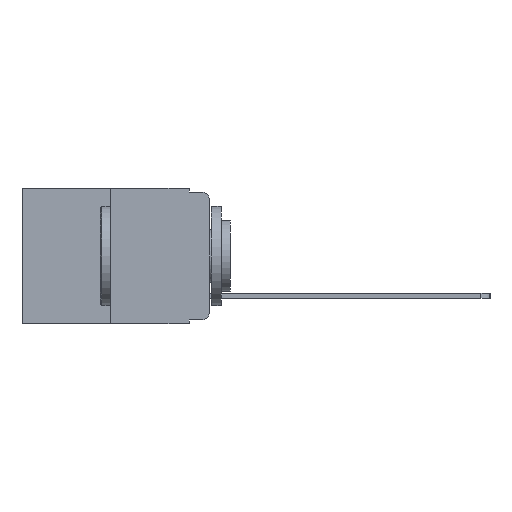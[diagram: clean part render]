
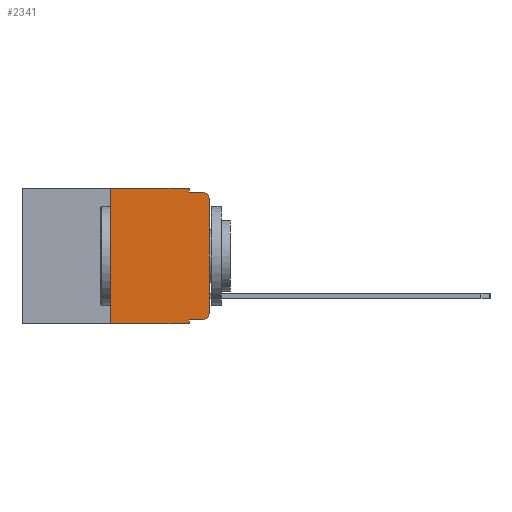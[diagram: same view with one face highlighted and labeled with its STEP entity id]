
A CAD part, left-side view. The second image highlights one B-rep face of the part: STEP entity #2341.
In plain terms, the highlighted planar face has unit normal (-1, 0, 0).
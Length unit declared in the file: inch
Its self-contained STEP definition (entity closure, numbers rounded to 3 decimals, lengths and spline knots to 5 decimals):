
#48 = CARTESIAN_POINT ( 'NONE',  ( 0., 0., -0.313 ) ) ;
#152 = LINE ( 'NONE', #20082, #4244 ) ;
#985 = CARTESIAN_POINT ( 'NONE',  ( 0., 0.25, 0. ) ) ;
#1154 = VERTEX_POINT ( 'NONE', #12719 ) ;
#1157 = EDGE_CURVE ( 'NONE', #9940, #8158, #12915, .T. ) ;
#1359 = VECTOR ( 'NONE', #15396, 39.37008 ) ;
#2341 = ADVANCED_FACE ( 'NONE', ( #12849 ), #18219, .F. ) ;
#2524 = ORIENTED_EDGE ( 'NONE', *, *, #1157, .T. ) ;
#2680 = DIRECTION ( 'NONE',  ( 0., -1., 0. ) ) ;
#2773 = EDGE_CURVE ( 'NONE', #5005, #10495, #17322, .T. ) ;
#3749 = ORIENTED_EDGE ( 'NONE', *, *, #14038, .F. ) ;
#3844 = VERTEX_POINT ( 'NONE', #15057 ) ;
#3892 = ORIENTED_EDGE ( 'NONE', *, *, #15682, .T. ) ;
#3919 = EDGE_LOOP ( 'NONE', ( #14781, #5084, #3749, #15264, #5722, #4393, #7224, #4700, #3892, #2524 ) ) ;
#4244 = VECTOR ( 'NONE', #7782, 39.37008 ) ;
#4262 = AXIS2_PLACEMENT_3D ( 'NONE', #7187, #18032, #8850 ) ;
#4393 = ORIENTED_EDGE ( 'NONE', *, *, #7287, .F. ) ;
#4700 = ORIENTED_EDGE ( 'NONE', *, *, #8414, .F. ) ;
#5005 = VERTEX_POINT ( 'NONE', #12021 ) ;
#5084 = ORIENTED_EDGE ( 'NONE', *, *, #20448, .T. ) ;
#5722 = ORIENTED_EDGE ( 'NONE', *, *, #17112, .F. ) ;
#6088 = LINE ( 'NONE', #13974, #17572 ) ;
#7130 = CARTESIAN_POINT ( 'NONE',  ( 0., 0.051, -0.01 ) ) ;
#7187 = CARTESIAN_POINT ( 'NONE',  ( 0., 0.02, -0.03 ) ) ;
#7224 = ORIENTED_EDGE ( 'NONE', *, *, #13374, .T. ) ;
#7287 = EDGE_CURVE ( 'NONE', #1154, #10195, #15985, .T. ) ;
#7782 = DIRECTION ( 'NONE',  ( 0., 0., -1. ) ) ;
#8158 = VERTEX_POINT ( 'NONE', #48 ) ;
#8163 = CARTESIAN_POINT ( 'NONE',  ( 0., 0., -0.03 ) ) ;
#8414 = EDGE_CURVE ( 'NONE', #10343, #12757, #152, .T. ) ;
#8566 = CARTESIAN_POINT ( 'NONE',  ( 0., 0.473, 0. ) ) ;
#8850 = DIRECTION ( 'NONE',  ( 0., 0., -1. ) ) ;
#9265 = VECTOR ( 'NONE', #10903, 39.37008 ) ;
#9369 = DIRECTION ( 'NONE',  ( 0., -1., 0. ) ) ;
#9417 = DIRECTION ( 'NONE',  ( 0., 0., -1. ) ) ;
#9788 = LINE ( 'NONE', #19992, #9265 ) ;
#9876 = VECTOR ( 'NONE', #9369, 39.37008 ) ;
#9940 = VERTEX_POINT ( 'NONE', #15331 ) ;
#10195 = VERTEX_POINT ( 'NONE', #15844 ) ;
#10343 = VERTEX_POINT ( 'NONE', #19184 ) ;
#10495 = VERTEX_POINT ( 'NONE', #7130 ) ;
#10903 = DIRECTION ( 'NONE',  ( 0., -1., 0. ) ) ;
#11580 = CARTESIAN_POINT ( 'NONE',  ( 0., 0., 0. ) ) ;
#11679 = DIRECTION ( 'NONE',  ( 0., 0., -1. ) ) ;
#11693 = CIRCLE ( 'NONE', #4262, 0.02 ) ;
#11727 = DIRECTION ( 'NONE',  ( -1., 0., 0. ) ) ;
#11831 = CARTESIAN_POINT ( 'NONE',  ( 0., 0.02, -0.313 ) ) ;
#12021 = CARTESIAN_POINT ( 'NONE',  ( 0., 0.051, 0. ) ) ;
#12719 = CARTESIAN_POINT ( 'NONE',  ( 0., 0.25, -0.343 ) ) ;
#12757 = VERTEX_POINT ( 'NONE', #14078 ) ;
#12785 = LINE ( 'NONE', #11580, #20310 ) ;
#12849 = FACE_OUTER_BOUND ( 'NONE', #3919, .T. ) ;
#12915 = CIRCLE ( 'NONE', #18375, 0.02 ) ;
#13107 = DIRECTION ( 'NONE',  ( 0., 0., 1. ) ) ;
#13288 = VECTOR ( 'NONE', #9417, 39.37008 ) ;
#13374 = EDGE_CURVE ( 'NONE', #1154, #12757, #9788, .T. ) ;
#13974 = CARTESIAN_POINT ( 'NONE',  ( 0., 0.051, -0.333 ) ) ;
#13985 = LINE ( 'NONE', #17030, #9876 ) ;
#14038 = EDGE_CURVE ( 'NONE', #10495, #3844, #18367, .T. ) ;
#14078 = CARTESIAN_POINT ( 'NONE',  ( 0., 0.051, -0.343 ) ) ;
#14287 = CARTESIAN_POINT ( 'NONE',  ( 0., 0.051, 0. ) ) ;
#14781 = ORIENTED_EDGE ( 'NONE', *, *, #17452, .T. ) ;
#15057 = CARTESIAN_POINT ( 'NONE',  ( 0., 0.02, -0.01 ) ) ;
#15131 = AXIS2_PLACEMENT_3D ( 'NONE', #8566, #20245, #15872 ) ;
#15264 = ORIENTED_EDGE ( 'NONE', *, *, #2773, .F. ) ;
#15331 = CARTESIAN_POINT ( 'NONE',  ( 0., 0.02, -0.333 ) ) ;
#15396 = DIRECTION ( 'NONE',  ( 0., -1., 0. ) ) ;
#15682 = EDGE_CURVE ( 'NONE', #10343, #9940, #6088, .T. ) ;
#15844 = CARTESIAN_POINT ( 'NONE',  ( 0., 0.25, 0. ) ) ;
#15872 = DIRECTION ( 'NONE',  ( 0., 0., -1. ) ) ;
#15985 = LINE ( 'NONE', #985, #16926 ) ;
#16926 = VECTOR ( 'NONE', #17066, 39.37008 ) ;
#17030 = CARTESIAN_POINT ( 'NONE',  ( 0., 0.473, 0. ) ) ;
#17066 = DIRECTION ( 'NONE',  ( 0., 0., 1. ) ) ;
#17112 = EDGE_CURVE ( 'NONE', #10195, #5005, #13985, .T. ) ;
#17318 = VERTEX_POINT ( 'NONE', #8163 ) ;
#17322 = LINE ( 'NONE', #14287, #13288 ) ;
#17452 = EDGE_CURVE ( 'NONE', #8158, #17318, #12785, .T. ) ;
#17572 = VECTOR ( 'NONE', #2680, 39.37008 ) ;
#18032 = DIRECTION ( 'NONE',  ( -1., 0., 0. ) ) ;
#18219 = PLANE ( 'NONE',  #15131 ) ;
#18367 = LINE ( 'NONE', #18411, #1359 ) ;
#18375 = AXIS2_PLACEMENT_3D ( 'NONE', #11831, #11727, #11679 ) ;
#18411 = CARTESIAN_POINT ( 'NONE',  ( 0., 0.051, -0.01 ) ) ;
#19184 = CARTESIAN_POINT ( 'NONE',  ( 0., 0.051, -0.333 ) ) ;
#19992 = CARTESIAN_POINT ( 'NONE',  ( 0., 0.473, -0.343 ) ) ;
#20082 = CARTESIAN_POINT ( 'NONE',  ( 0., 0.051, 0. ) ) ;
#20245 = DIRECTION ( 'NONE',  ( 1., 0., 0. ) ) ;
#20310 = VECTOR ( 'NONE', #13107, 39.37008 ) ;
#20448 = EDGE_CURVE ( 'NONE', #17318, #3844, #11693, .T. ) ;
